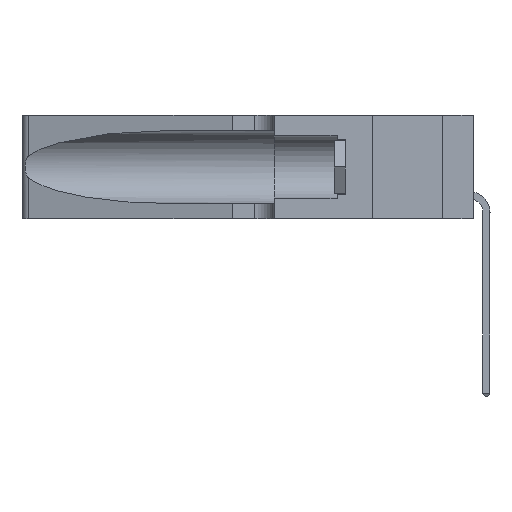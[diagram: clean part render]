
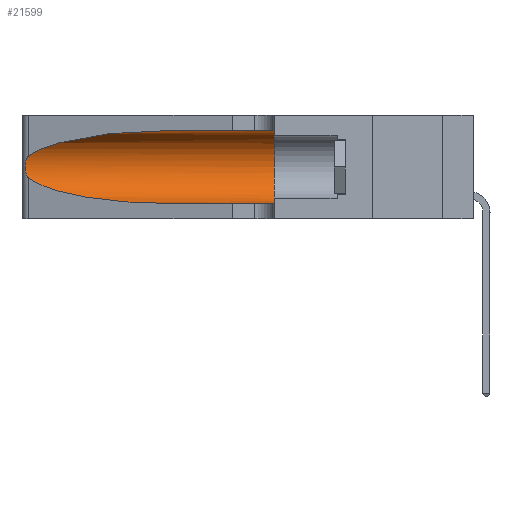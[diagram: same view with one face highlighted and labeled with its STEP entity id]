
A CAD part, left-side view. The second image highlights one B-rep face of the part: STEP entity #21599.
In plain terms, the highlighted cylindrical face has radius 3.308 mm (diameter 6.617 mm), a partial arc.
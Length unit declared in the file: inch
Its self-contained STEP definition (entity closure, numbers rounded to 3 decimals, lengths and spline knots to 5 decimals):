
#272 = CIRCLE ( 'NONE', #11519, 0.13025 ) ;
#494 = VERTEX_POINT ( 'NONE', #4612 ) ;
#1216 = DIRECTION ( 'NONE',  ( 0., 0., 1. ) ) ;
#1374 = CARTESIAN_POINT ( 'NONE',  ( 0.18966, 0.96281, 0.31525 ) ) ;
#1591 = CARTESIAN_POINT ( 'NONE',  ( 0.25555, 1.22993, 0.14849 ) ) ;
#1797 = AXIS2_PLACEMENT_3D ( 'NONE', #2901, #2195, #19791 ) ;
#2195 = DIRECTION ( 'NONE',  ( 0., -1., 0. ) ) ;
#2901 = CARTESIAN_POINT ( 'NONE',  ( 0.1305, 1.61858, 0.185 ) ) ;
#3364 = VERTEX_POINT ( 'NONE', #16597 ) ;
#4612 = CARTESIAN_POINT ( 'NONE',  ( 0.1305, 0.72297, 0.31525 ) ) ;
#5168 = VECTOR ( 'NONE', #17647, 39.37008 ) ;
#5891 = ORIENTED_EDGE ( 'NONE', *, *, #15127, .T. ) ;
#6225 = FACE_OUTER_BOUND ( 'NONE', #16674, .T. ) ;
#6440 = B_SPLINE_CURVE_WITH_KNOTS ( 'NONE', 3,
 ( #22901, #15373, #15289, #21307, #9479, #17095, #13153, #9311, #22986, #13319, #11258, #17343, #1591, #9568 ),
 .UNSPECIFIED., .F., .F.,
 ( 4, 2, 2, 2, 2, 2, 4 ),
 ( 0., 0.00027, 0.00053, 0.00107, 0.0016, 0.00187, 0.00214 ),
 .UNSPECIFIED. ) ;
#6466 = EDGE_CURVE ( 'NONE', #8930, #3364, #16982, .T. ) ;
#7135 = CARTESIAN_POINT ( 'NONE',  ( 0.1305, 0.72297, 0.31525 ) ) ;
#8096 = DIRECTION ( 'NONE',  ( 0., -1., 0. ) ) ;
#8239 = ORIENTED_EDGE ( 'NONE', *, *, #10500, .T. ) ;
#8299 = EDGE_CURVE ( 'NONE', #494, #20757, #23825, .T. ) ;
#8328 = CARTESIAN_POINT ( 'NONE',  ( 0.25487, 1.22718, 0.14631 ) ) ;
#8930 = VERTEX_POINT ( 'NONE', #18324 ) ;
#9013 = CARTESIAN_POINT ( 'NONE',  ( 0.1305, 0.35, 0.185 ) ) ;
#9311 = CARTESIAN_POINT ( 'NONE',  ( 0.26075, 1.23896, 0.178 ) ) ;
#9479 = CARTESIAN_POINT ( 'NONE',  ( 0.25854, 1.2359, 0.20912 ) ) ;
#9568 = CARTESIAN_POINT ( 'NONE',  ( 0.25487, 1.22718, 0.14631 ) ) ;
#10076 = VECTOR ( 'NONE', #8096, 39.37008 ) ;
#10299 = CARTESIAN_POINT ( 'NONE',  ( 0.18966, 0.96281, 0.05475 ) ) ;
#10500 = EDGE_CURVE ( 'NONE', #494, #20486, #14443, .T. ) ;
#10907 = CARTESIAN_POINT ( 'NONE',  ( 0.1305, 0.35, 0.05475 ) ) ;
#10964 = CARTESIAN_POINT ( 'NONE',  ( 0.1305, 0.35, 0.31525 ) ) ;
#11258 = CARTESIAN_POINT ( 'NONE',  ( 0.25789, 1.23486, 0.15765 ) ) ;
#11519 = AXIS2_PLACEMENT_3D ( 'NONE', #9013, #20625, #1216 ) ;
#11871 = LINE ( 'NONE', #21617, #10076 ) ;
#12285 = ORIENTED_EDGE ( 'NONE', *, *, #15968, .F. ) ;
#13153 = CARTESIAN_POINT ( 'NONE',  ( 0.26075, 1.23896, 0.19203 ) ) ;
#13319 = CARTESIAN_POINT ( 'NONE',  ( 0.25856, 1.23593, 0.16098 ) ) ;
#14443 =( BOUNDED_CURVE ( )  B_SPLINE_CURVE ( 3, ( #7135, #1374, #20796, #17210 ),
 .UNSPECIFIED., .F., .T. ) 
 B_SPLINE_CURVE_WITH_KNOTS ( ( 4, 4 ),
 ( 1.5708, 2.84003 ),
 .UNSPECIFIED. ) 
 CURVE ( )  GEOMETRIC_REPRESENTATION_ITEM ( )  RATIONAL_B_SPLINE_CURVE ( ( 1., 0.87, 0.87, 1. ) ) 
 REPRESENTATION_ITEM ( '' )  );
#14778 = EDGE_CURVE ( 'NONE', #20486, #8930, #6440, .T. ) ;
#14786 = CYLINDRICAL_SURFACE ( 'NONE', #1797, 0.13025 ) ;
#15127 = EDGE_CURVE ( 'NONE', #3364, #22211, #11871, .T. ) ;
#15289 = CARTESIAN_POINT ( 'NONE',  ( 0.25639, 1.23184, 0.21858 ) ) ;
#15373 = CARTESIAN_POINT ( 'NONE',  ( 0.25555, 1.22994, 0.2215 ) ) ;
#15968 = EDGE_CURVE ( 'NONE', #20757, #22211, #272, .T. ) ;
#16278 = CARTESIAN_POINT ( 'NONE',  ( 0.2373, 1.15595, 0.08982 ) ) ;
#16597 = CARTESIAN_POINT ( 'NONE',  ( 0.1305, 0.72297, 0.05475 ) ) ;
#16674 = EDGE_LOOP ( 'NONE', ( #8239, #19017, #23066, #5891, #12285, #23796 ) ) ;
#16982 =( BOUNDED_CURVE ( )  B_SPLINE_CURVE ( 3, ( #8328, #16278, #10299, #22260 ),
 .UNSPECIFIED., .F., .T. ) 
 B_SPLINE_CURVE_WITH_KNOTS ( ( 4, 4 ),
 ( 3.44316, 4.71239 ),
 .UNSPECIFIED. ) 
 CURVE ( )  GEOMETRIC_REPRESENTATION_ITEM ( )  RATIONAL_B_SPLINE_CURVE ( ( 1., 0.87, 0.87, 1. ) ) 
 REPRESENTATION_ITEM ( '' )  );
#17095 = CARTESIAN_POINT ( 'NONE',  ( 0.26018, 1.23835, 0.19895 ) ) ;
#17210 = CARTESIAN_POINT ( 'NONE',  ( 0.25487, 1.22718, 0.22369 ) ) ;
#17343 = CARTESIAN_POINT ( 'NONE',  ( 0.25639, 1.23186, 0.15144 ) ) ;
#17647 = DIRECTION ( 'NONE',  ( 0., -1., 0. ) ) ;
#18324 = CARTESIAN_POINT ( 'NONE',  ( 0.25487, 1.22718, 0.14631 ) ) ;
#19017 = ORIENTED_EDGE ( 'NONE', *, *, #14778, .T. ) ;
#19791 = DIRECTION ( 'NONE',  ( 0., 0., -1. ) ) ;
#20486 = VERTEX_POINT ( 'NONE', #21749 ) ;
#20625 = DIRECTION ( 'NONE',  ( 0., 1., 0. ) ) ;
#20757 = VERTEX_POINT ( 'NONE', #10964 ) ;
#20796 = CARTESIAN_POINT ( 'NONE',  ( 0.2373, 1.15595, 0.28018 ) ) ;
#21307 = CARTESIAN_POINT ( 'NONE',  ( 0.25787, 1.23484, 0.2124 ) ) ;
#21592 = CARTESIAN_POINT ( 'NONE',  ( 0.1305, 1.61858, 0.31525 ) ) ;
#21599 = ADVANCED_FACE ( 'NONE', ( #6225 ), #14786, .F. ) ;
#21617 = CARTESIAN_POINT ( 'NONE',  ( 0.1305, 1.61858, 0.05475 ) ) ;
#21749 = CARTESIAN_POINT ( 'NONE',  ( 0.25487, 1.22718, 0.22369 ) ) ;
#22211 = VERTEX_POINT ( 'NONE', #10907 ) ;
#22260 = CARTESIAN_POINT ( 'NONE',  ( 0.1305, 0.72297, 0.05475 ) ) ;
#22901 = CARTESIAN_POINT ( 'NONE',  ( 0.25487, 1.22718, 0.22369 ) ) ;
#22986 = CARTESIAN_POINT ( 'NONE',  ( 0.26017, 1.23833, 0.17102 ) ) ;
#23066 = ORIENTED_EDGE ( 'NONE', *, *, #6466, .T. ) ;
#23796 = ORIENTED_EDGE ( 'NONE', *, *, #8299, .F. ) ;
#23825 = LINE ( 'NONE', #21592, #5168 ) ;
